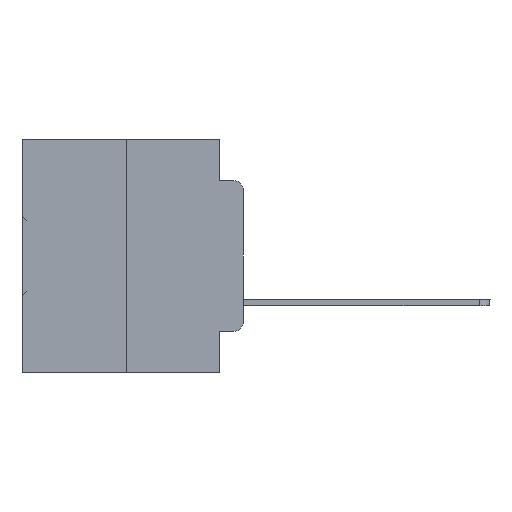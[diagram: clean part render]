
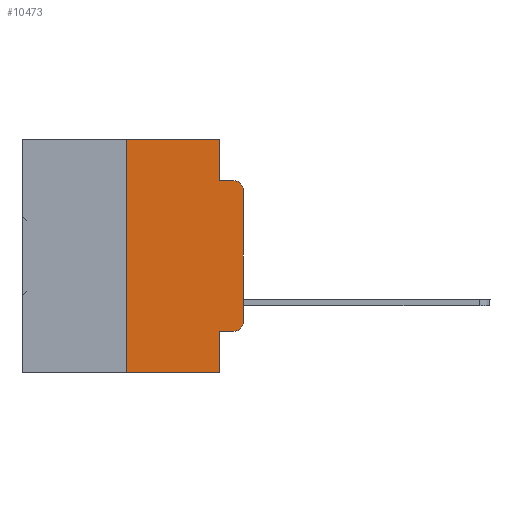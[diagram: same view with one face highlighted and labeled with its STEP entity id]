
A CAD part, left-side view. The second image highlights one B-rep face of the part: STEP entity #10473.
In plain terms, the highlighted planar face has unit normal (-1, 0, 0).
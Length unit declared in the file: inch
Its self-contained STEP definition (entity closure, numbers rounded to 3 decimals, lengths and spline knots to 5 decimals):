
#313 = CARTESIAN_POINT ( 'NONE',  ( 0., 0.02, -0.1085 ) ) ;
#550 = CARTESIAN_POINT ( 'NONE',  ( 0., 0.02, -0.0885 ) ) ;
#2134 = DIRECTION ( 'NONE',  ( 0., 0., -1. ) ) ;
#2624 = CARTESIAN_POINT ( 'NONE',  ( 0., 0.051, 0. ) ) ;
#2803 = EDGE_CURVE ( 'NONE', #12834, #30827, #20056, .T. ) ;
#3353 = DIRECTION ( 'NONE',  ( 0., -1., 0. ) ) ;
#3454 = CARTESIAN_POINT ( 'NONE',  ( 0., 0.25, 0. ) ) ;
#3954 = ORIENTED_EDGE ( 'NONE', *, *, #7065, .T. ) ;
#4159 = VERTEX_POINT ( 'NONE', #550 ) ;
#4932 = CARTESIAN_POINT ( 'NONE',  ( 0., 0.25, 0. ) ) ;
#5030 = CARTESIAN_POINT ( 'NONE',  ( 0., 0.051, 0. ) ) ;
#5050 = VECTOR ( 'NONE', #28779, 39.37008 ) ;
#6067 = EDGE_CURVE ( 'NONE', #12834, #30091, #15105, .T. ) ;
#6723 = CARTESIAN_POINT ( 'NONE',  ( 0., 0.02, -0.4115 ) ) ;
#7014 = VECTOR ( 'NONE', #27263, 39.37008 ) ;
#7065 = EDGE_CURVE ( 'NONE', #8571, #4159, #26606, .T. ) ;
#7077 = DIRECTION ( 'NONE',  ( 0., 0., -1. ) ) ;
#7122 = LINE ( 'NONE', #28986, #15500 ) ;
#8036 = DIRECTION ( 'NONE',  ( 0., 0., 1. ) ) ;
#8130 = VECTOR ( 'NONE', #3353, 39.37008 ) ;
#8571 = VERTEX_POINT ( 'NONE', #8763 ) ;
#8763 = CARTESIAN_POINT ( 'NONE',  ( 0., 0., -0.1085 ) ) ;
#9596 = CARTESIAN_POINT ( 'NONE',  ( 0., 0.051, -0.5 ) ) ;
#9834 = CARTESIAN_POINT ( 'NONE',  ( 0., 0.25, -0.5 ) ) ;
#10192 = DIRECTION ( 'NONE',  ( 0., -1., 0. ) ) ;
#10473 = ADVANCED_FACE ( 'NONE', ( #13051 ), #29483, .F. ) ;
#11084 = VERTEX_POINT ( 'NONE', #2624 ) ;
#11204 = EDGE_CURVE ( 'NONE', #28464, #32043, #30927, .T. ) ;
#11711 = VERTEX_POINT ( 'NONE', #25403 ) ;
#11737 = ORIENTED_EDGE ( 'NONE', *, *, #2803, .T. ) ;
#12330 = CARTESIAN_POINT ( 'NONE',  ( 0., 0., -0.3915 ) ) ;
#12494 = EDGE_CURVE ( 'NONE', #11711, #30827, #33332, .T. ) ;
#12834 = VERTEX_POINT ( 'NONE', #9834 ) ;
#13051 = FACE_OUTER_BOUND ( 'NONE', #25677, .T. ) ;
#13350 = ORIENTED_EDGE ( 'NONE', *, *, #18145, .F. ) ;
#13561 = ORIENTED_EDGE ( 'NONE', *, *, #23780, .T. ) ;
#14449 = CARTESIAN_POINT ( 'NONE',  ( 0., 0.051, -0.4115 ) ) ;
#15105 = LINE ( 'NONE', #3454, #5050 ) ;
#15500 = VECTOR ( 'NONE', #10192, 39.37008 ) ;
#15801 = DIRECTION ( 'NONE',  ( 1., 0., 0. ) ) ;
#16477 = LINE ( 'NONE', #5030, #7014 ) ;
#16981 = VECTOR ( 'NONE', #30076, 39.37008 ) ;
#17325 = DIRECTION ( 'NONE',  ( 0., -1., 0. ) ) ;
#18054 = LINE ( 'NONE', #21329, #30709 ) ;
#18145 = EDGE_CURVE ( 'NONE', #30091, #11084, #7122, .T. ) ;
#19753 = LINE ( 'NONE', #14449, #8130 ) ;
#19995 = ORIENTED_EDGE ( 'NONE', *, *, #27958, .F. ) ;
#20056 = LINE ( 'NONE', #31172, #32454 ) ;
#20541 = ORIENTED_EDGE ( 'NONE', *, *, #22835, .T. ) ;
#20973 = DIRECTION ( 'NONE',  ( 0., -1., 0. ) ) ;
#21280 = CARTESIAN_POINT ( 'NONE',  ( 0., 0.473, 0. ) ) ;
#21329 = CARTESIAN_POINT ( 'NONE',  ( 0., 0.051, -0.0885 ) ) ;
#21622 = AXIS2_PLACEMENT_3D ( 'NONE', #35274, #23646, #7077 ) ;
#22144 = AXIS2_PLACEMENT_3D ( 'NONE', #21280, #15801, #2134 ) ;
#22359 = DIRECTION ( 'NONE',  ( 0., 0., -1. ) ) ;
#22835 = EDGE_CURVE ( 'NONE', #11711, #28464, #19753, .T. ) ;
#23646 = DIRECTION ( 'NONE',  ( -1., 0., 0. ) ) ;
#23780 = EDGE_CURVE ( 'NONE', #32043, #8571, #35705, .T. ) ;
#25075 = ORIENTED_EDGE ( 'NONE', *, *, #12494, .F. ) ;
#25403 = CARTESIAN_POINT ( 'NONE',  ( 0., 0.051, -0.4115 ) ) ;
#25677 = EDGE_LOOP ( 'NONE', ( #13561, #3954, #19995, #26574, #13350, #32029, #11737, #25075, #20541, #32106 ) ) ;
#26574 = ORIENTED_EDGE ( 'NONE', *, *, #32329, .F. ) ;
#26606 = CIRCLE ( 'NONE', #35313, 0.02 ) ;
#26818 = VECTOR ( 'NONE', #8036, 39.37008 ) ;
#27263 = DIRECTION ( 'NONE',  ( 0., 0., -1. ) ) ;
#27958 = EDGE_CURVE ( 'NONE', #33049, #4159, #18054, .T. ) ;
#28464 = VERTEX_POINT ( 'NONE', #6723 ) ;
#28779 = DIRECTION ( 'NONE',  ( 0., 0., 1. ) ) ;
#28986 = CARTESIAN_POINT ( 'NONE',  ( 0., 0.473, 0. ) ) ;
#29027 = CARTESIAN_POINT ( 'NONE',  ( 0., 0.051, -0.0885 ) ) ;
#29483 = PLANE ( 'NONE',  #22144 ) ;
#30076 = DIRECTION ( 'NONE',  ( 0., 0., -1. ) ) ;
#30091 = VERTEX_POINT ( 'NONE', #4932 ) ;
#30709 = VECTOR ( 'NONE', #20973, 39.37008 ) ;
#30827 = VERTEX_POINT ( 'NONE', #9596 ) ;
#30927 = CIRCLE ( 'NONE', #21622, 0.02 ) ;
#31172 = CARTESIAN_POINT ( 'NONE',  ( 0., 0.473, -0.5 ) ) ;
#32029 = ORIENTED_EDGE ( 'NONE', *, *, #6067, .F. ) ;
#32043 = VERTEX_POINT ( 'NONE', #12330 ) ;
#32106 = ORIENTED_EDGE ( 'NONE', *, *, #11204, .T. ) ;
#32329 = EDGE_CURVE ( 'NONE', #11084, #33049, #16477, .T. ) ;
#32454 = VECTOR ( 'NONE', #17325, 39.37008 ) ;
#32748 = DIRECTION ( 'NONE',  ( -1., 0., 0. ) ) ;
#32983 = CARTESIAN_POINT ( 'NONE',  ( 0., 0.051, 0. ) ) ;
#32993 = CARTESIAN_POINT ( 'NONE',  ( 0., 0., 0. ) ) ;
#33049 = VERTEX_POINT ( 'NONE', #29027 ) ;
#33332 = LINE ( 'NONE', #32983, #16981 ) ;
#35274 = CARTESIAN_POINT ( 'NONE',  ( 0., 0.02, -0.3915 ) ) ;
#35313 = AXIS2_PLACEMENT_3D ( 'NONE', #313, #32748, #22359 ) ;
#35705 = LINE ( 'NONE', #32993, #26818 ) ;
